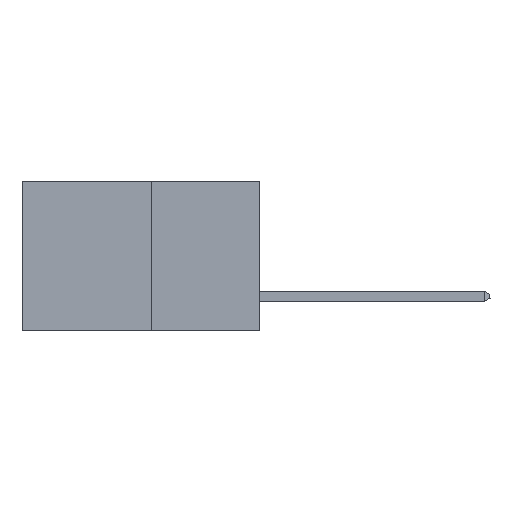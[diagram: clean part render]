
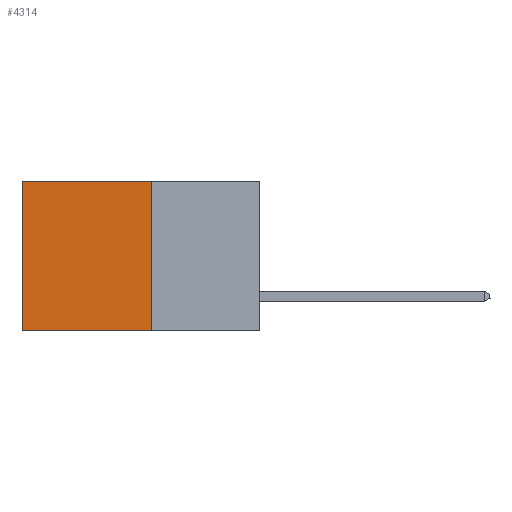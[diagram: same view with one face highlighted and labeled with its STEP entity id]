
A CAD part, left-side view. The second image highlights one B-rep face of the part: STEP entity #4314.
In plain terms, the highlighted planar face has unit normal (-1, 0, 0).
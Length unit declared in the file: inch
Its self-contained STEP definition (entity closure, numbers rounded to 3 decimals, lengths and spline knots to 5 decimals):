
#749 = EDGE_CURVE ( 'NONE', #9120, #14010, #9313, .T. ) ;
#953 = VECTOR ( 'NONE', #5716, 39.37008 ) ;
#1763 = FACE_OUTER_BOUND ( 'NONE', #6357, .T. ) ;
#2260 = PLANE ( 'NONE',  #12903 ) ;
#2449 = DIRECTION ( 'NONE',  ( 0., 0., -1. ) ) ;
#2505 = DIRECTION ( 'NONE',  ( 1., 0., 0. ) ) ;
#2976 = LINE ( 'NONE', #12655, #8472 ) ;
#3086 = EDGE_CURVE ( 'NONE', #7573, #14010, #2976, .T. ) ;
#3648 = CARTESIAN_POINT ( 'NONE',  ( 0.277, 0.27, -0.37 ) ) ;
#3664 = CARTESIAN_POINT ( 'NONE',  ( 0.277, 0.59, 0. ) ) ;
#3846 = CARTESIAN_POINT ( 'NONE',  ( 0.277, 0.27, -0.37 ) ) ;
#3941 = ORIENTED_EDGE ( 'NONE', *, *, #3086, .F. ) ;
#4314 = ADVANCED_FACE ( 'NONE', ( #1763 ), #2260, .F. ) ;
#4480 = ORIENTED_EDGE ( 'NONE', *, *, #10798, .F. ) ;
#4624 = CARTESIAN_POINT ( 'NONE',  ( 0.277, 0.59, -0.37 ) ) ;
#5062 = EDGE_CURVE ( 'NONE', #7403, #9120, #5291, .T. ) ;
#5291 = LINE ( 'NONE', #13598, #10717 ) ;
#5704 = CARTESIAN_POINT ( 'NONE',  ( 0.277, 0.27, 0. ) ) ;
#5716 = DIRECTION ( 'NONE',  ( 0., 0., -1. ) ) ;
#6357 = EDGE_LOOP ( 'NONE', ( #12199, #3941, #4480, #7179 ) ) ;
#6504 = DIRECTION ( 'NONE',  ( 0., 0., -1. ) ) ;
#7179 = ORIENTED_EDGE ( 'NONE', *, *, #5062, .T. ) ;
#7386 = VECTOR ( 'NONE', #6504, 39.37008 ) ;
#7403 = VERTEX_POINT ( 'NONE', #5704 ) ;
#7573 = VERTEX_POINT ( 'NONE', #3846 ) ;
#8472 = VECTOR ( 'NONE', #10377, 39.37008 ) ;
#9120 = VERTEX_POINT ( 'NONE', #3664 ) ;
#9313 = LINE ( 'NONE', #10313, #953 ) ;
#10313 = CARTESIAN_POINT ( 'NONE',  ( 0.277, 0.59, -0.37 ) ) ;
#10377 = DIRECTION ( 'NONE',  ( 0., 1., 0. ) ) ;
#10717 = VECTOR ( 'NONE', #13544, 39.37008 ) ;
#10798 = EDGE_CURVE ( 'NONE', #7403, #7573, #13020, .T. ) ;
#12199 = ORIENTED_EDGE ( 'NONE', *, *, #749, .T. ) ;
#12655 = CARTESIAN_POINT ( 'NONE',  ( 0.277, 0.27, -0.37 ) ) ;
#12903 = AXIS2_PLACEMENT_3D ( 'NONE', #3648, #2505, #2449 ) ;
#12927 = CARTESIAN_POINT ( 'NONE',  ( 0.277, 0.27, -0.37 ) ) ;
#13020 = LINE ( 'NONE', #12927, #7386 ) ;
#13544 = DIRECTION ( 'NONE',  ( 0., 1., 0. ) ) ;
#13598 = CARTESIAN_POINT ( 'NONE',  ( 0.277, 0.27, 0. ) ) ;
#14010 = VERTEX_POINT ( 'NONE', #4624 ) ;
